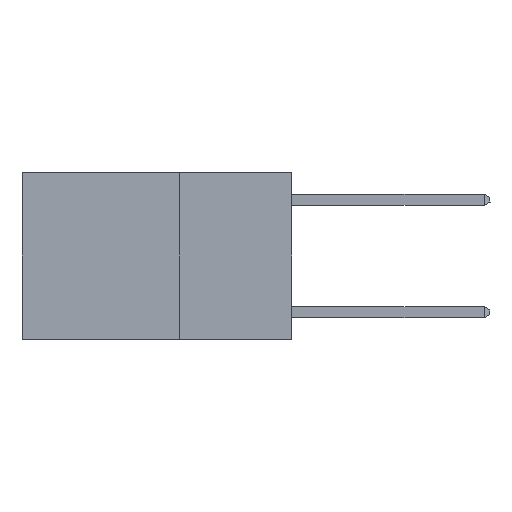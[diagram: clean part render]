
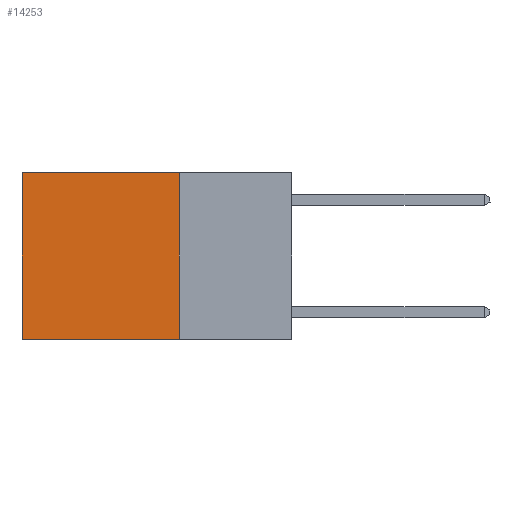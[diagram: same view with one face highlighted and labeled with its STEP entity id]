
A CAD part, left-side view. The second image highlights one B-rep face of the part: STEP entity #14253.
In plain terms, the highlighted planar face has unit normal (-1, 0, 0).
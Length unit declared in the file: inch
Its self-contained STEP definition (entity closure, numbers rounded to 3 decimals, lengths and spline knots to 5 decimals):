
#319 = VERTEX_POINT ( 'NONE', #3195 ) ;
#519 = PLANE ( 'NONE',  #5454 ) ;
#1023 = EDGE_CURVE ( 'NONE', #7310, #14937, #10933, .T. ) ;
#1564 = CARTESIAN_POINT ( 'NONE',  ( 0.2625, 0.25, 0. ) ) ;
#1746 = ORIENTED_EDGE ( 'NONE', *, *, #14590, .F. ) ;
#1819 = VERTEX_POINT ( 'NONE', #8787 ) ;
#1866 = CARTESIAN_POINT ( 'NONE',  ( 0.2625, 0.25, 0. ) ) ;
#1871 = DIRECTION ( 'NONE',  ( 1., 0., 0. ) ) ;
#3195 = CARTESIAN_POINT ( 'NONE',  ( 0.2625, 0.6, -0.37 ) ) ;
#4061 = VECTOR ( 'NONE', #12263, 39.37008 ) ;
#4956 = DIRECTION ( 'NONE',  ( 0., 0., -1. ) ) ;
#5061 = LINE ( 'NONE', #16618, #14873 ) ;
#5445 = LINE ( 'NONE', #8064, #8853 ) ;
#5454 = AXIS2_PLACEMENT_3D ( 'NONE', #9660, #1871, #10964 ) ;
#5481 = DIRECTION ( 'NONE',  ( 0., 0., -1. ) ) ;
#6913 = FACE_OUTER_BOUND ( 'NONE', #10851, .T. ) ;
#7310 = VERTEX_POINT ( 'NONE', #1564 ) ;
#8064 = CARTESIAN_POINT ( 'NONE',  ( 0.2625, 0.6, 0. ) ) ;
#8787 = CARTESIAN_POINT ( 'NONE',  ( 0.2625, 0.25, -0.37 ) ) ;
#8853 = VECTOR ( 'NONE', #5481, 39.37008 ) ;
#9660 = CARTESIAN_POINT ( 'NONE',  ( 0.2625, 0.25, 0. ) ) ;
#9749 = CARTESIAN_POINT ( 'NONE',  ( 0.2625, 0.6, 0. ) ) ;
#9911 = LINE ( 'NONE', #16375, #16251 ) ;
#10851 = EDGE_LOOP ( 'NONE', ( #16499, #1746, #11194, #16613 ) ) ;
#10933 = LINE ( 'NONE', #1866, #4061 ) ;
#10964 = DIRECTION ( 'NONE',  ( 0., 0., -1. ) ) ;
#11194 = ORIENTED_EDGE ( 'NONE', *, *, #13817, .F. ) ;
#11630 = DIRECTION ( 'NONE',  ( 0., 1., 0. ) ) ;
#12263 = DIRECTION ( 'NONE',  ( 0., 1., 0. ) ) ;
#13817 = EDGE_CURVE ( 'NONE', #7310, #1819, #9911, .T. ) ;
#14253 = ADVANCED_FACE ( 'NONE', ( #6913 ), #519, .F. ) ;
#14590 = EDGE_CURVE ( 'NONE', #1819, #319, #5061, .T. ) ;
#14873 = VECTOR ( 'NONE', #11630, 39.37008 ) ;
#14937 = VERTEX_POINT ( 'NONE', #9749 ) ;
#15355 = EDGE_CURVE ( 'NONE', #14937, #319, #5445, .T. ) ;
#16251 = VECTOR ( 'NONE', #4956, 39.37008 ) ;
#16375 = CARTESIAN_POINT ( 'NONE',  ( 0.2625, 0.25, 0. ) ) ;
#16499 = ORIENTED_EDGE ( 'NONE', *, *, #15355, .T. ) ;
#16613 = ORIENTED_EDGE ( 'NONE', *, *, #1023, .T. ) ;
#16618 = CARTESIAN_POINT ( 'NONE',  ( 0.2625, 0.25, -0.37 ) ) ;
